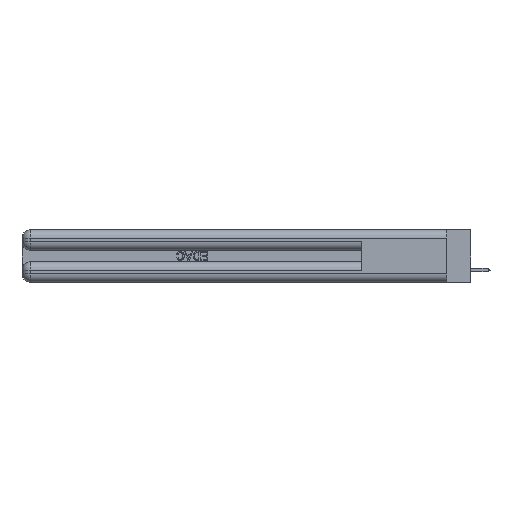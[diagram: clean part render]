
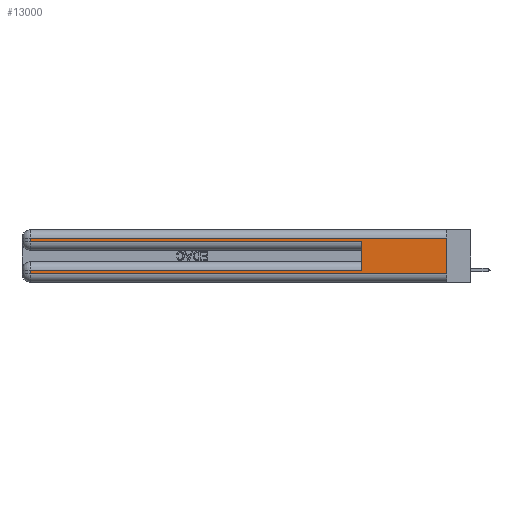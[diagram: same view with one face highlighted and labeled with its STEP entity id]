
A CAD part, left-side view. The second image highlights one B-rep face of the part: STEP entity #13000.
In plain terms, the highlighted planar face has unit normal (-1, 0, 0).
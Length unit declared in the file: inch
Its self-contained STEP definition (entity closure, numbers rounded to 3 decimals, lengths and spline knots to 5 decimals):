
#81 = ORIENTED_EDGE ( 'NONE', *, *, #29845, .T. ) ;
#892 = EDGE_LOOP ( 'NONE', ( #8477, #81, #23279, #6880, #42498, #15055, #4642, #9860 ) ) ;
#2024 = CARTESIAN_POINT ( 'NONE',  ( 0., 0., 0.085 ) ) ;
#2395 = CARTESIAN_POINT ( 'NONE',  ( 0., 2.94, 0.37 ) ) ;
#2813 = DIRECTION ( 'NONE',  ( 0., 0., -1. ) ) ;
#3315 = EDGE_CURVE ( 'NONE', #30173, #13856, #27101, .T. ) ;
#3468 = VECTOR ( 'NONE', #44397, 39.37008 ) ;
#4642 = ORIENTED_EDGE ( 'NONE', *, *, #40143, .T. ) ;
#6114 = LINE ( 'NONE', #21808, #14335 ) ;
#6879 = VERTEX_POINT ( 'NONE', #12419 ) ;
#6880 = ORIENTED_EDGE ( 'NONE', *, *, #42043, .T. ) ;
#7465 = AXIS2_PLACEMENT_3D ( 'NONE', #35042, #13983, #31778 ) ;
#7530 = VERTEX_POINT ( 'NONE', #21497 ) ;
#7731 = FACE_OUTER_BOUND ( 'NONE', #892, .T. ) ;
#8477 = ORIENTED_EDGE ( 'NONE', *, *, #14296, .F. ) ;
#8882 = LINE ( 'NONE', #28672, #34735 ) ;
#9617 = CARTESIAN_POINT ( 'NONE',  ( 0., 0., 0.37 ) ) ;
#9860 = ORIENTED_EDGE ( 'NONE', *, *, #44880, .T. ) ;
#10630 = CARTESIAN_POINT ( 'NONE',  ( 0., 0., 0.31 ) ) ;
#10912 = LINE ( 'NONE', #16637, #25170 ) ;
#11363 = DIRECTION ( 'NONE',  ( 0., 1., 0. ) ) ;
#12179 = CARTESIAN_POINT ( 'NONE',  ( 0., 2.94, 0.37 ) ) ;
#12419 = CARTESIAN_POINT ( 'NONE',  ( 0., 2.94, 0.06 ) ) ;
#13000 = ADVANCED_FACE ( 'NONE', ( #7731 ), #27669, .F. ) ;
#13856 = VERTEX_POINT ( 'NONE', #17220 ) ;
#13983 = DIRECTION ( 'NONE',  ( 1., 0., 0. ) ) ;
#14296 = EDGE_CURVE ( 'NONE', #29142, #7530, #25715, .T. ) ;
#14335 = VECTOR ( 'NONE', #11363, 39.37008 ) ;
#15055 = ORIENTED_EDGE ( 'NONE', *, *, #3315, .T. ) ;
#15820 = VECTOR ( 'NONE', #2813, 39.37008 ) ;
#16637 = CARTESIAN_POINT ( 'NONE',  ( 0., 0., 0.06 ) ) ;
#16802 = LINE ( 'NONE', #20202, #37574 ) ;
#17220 = CARTESIAN_POINT ( 'NONE',  ( 0., 2.94, 0.085 ) ) ;
#18384 = DIRECTION ( 'NONE',  ( 0., 0., 1. ) ) ;
#20202 = CARTESIAN_POINT ( 'NONE',  ( 0., 0., 0.285 ) ) ;
#20359 = DIRECTION ( 'NONE',  ( 0., 0., -1. ) ) ;
#21222 = VERTEX_POINT ( 'NONE', #44408 ) ;
#21497 = CARTESIAN_POINT ( 'NONE',  ( 0., 0., 0.06 ) ) ;
#21632 = EDGE_CURVE ( 'NONE', #30173, #21222, #8882, .T. ) ;
#21808 = CARTESIAN_POINT ( 'NONE',  ( 0., 0., 0.31 ) ) ;
#23279 = ORIENTED_EDGE ( 'NONE', *, *, #43675, .T. ) ;
#25148 = CARTESIAN_POINT ( 'NONE',  ( 0., 0.6, 0.085 ) ) ;
#25170 = VECTOR ( 'NONE', #30914, 39.37008 ) ;
#25715 = LINE ( 'NONE', #9617, #15820 ) ;
#26306 = DIRECTION ( 'NONE',  ( 0., 1., 0. ) ) ;
#26422 = VERTEX_POINT ( 'NONE', #34368 ) ;
#27101 = LINE ( 'NONE', #2024, #29225 ) ;
#27669 = PLANE ( 'NONE',  #7465 ) ;
#28672 = CARTESIAN_POINT ( 'NONE',  ( 0., 0.6, 0.145 ) ) ;
#29142 = VERTEX_POINT ( 'NONE', #10630 ) ;
#29225 = VECTOR ( 'NONE', #26306, 39.37008 ) ;
#29845 = EDGE_CURVE ( 'NONE', #29142, #26422, #6114, .T. ) ;
#30173 = VERTEX_POINT ( 'NONE', #25148 ) ;
#30914 = DIRECTION ( 'NONE',  ( 0., -1., 0. ) ) ;
#31778 = DIRECTION ( 'NONE',  ( 0., 0., -1. ) ) ;
#31917 = VECTOR ( 'NONE', #20359, 39.37008 ) ;
#34368 = CARTESIAN_POINT ( 'NONE',  ( 0., 2.94, 0.31 ) ) ;
#34735 = VECTOR ( 'NONE', #18384, 39.37008 ) ;
#34869 = LINE ( 'NONE', #2395, #3468 ) ;
#35042 = CARTESIAN_POINT ( 'NONE',  ( 0., 0., 0.37 ) ) ;
#35536 = VERTEX_POINT ( 'NONE', #35828 ) ;
#35828 = CARTESIAN_POINT ( 'NONE',  ( 0., 2.94, 0.285 ) ) ;
#37574 = VECTOR ( 'NONE', #41447, 39.37008 ) ;
#40143 = EDGE_CURVE ( 'NONE', #13856, #6879, #34869, .T. ) ;
#41447 = DIRECTION ( 'NONE',  ( 0., -1., 0. ) ) ;
#42043 = EDGE_CURVE ( 'NONE', #35536, #21222, #16802, .T. ) ;
#42498 = ORIENTED_EDGE ( 'NONE', *, *, #21632, .F. ) ;
#43482 = LINE ( 'NONE', #12179, #31917 ) ;
#43675 = EDGE_CURVE ( 'NONE', #26422, #35536, #43482, .T. ) ;
#44397 = DIRECTION ( 'NONE',  ( 0., 0., -1. ) ) ;
#44408 = CARTESIAN_POINT ( 'NONE',  ( 0., 0.6, 0.285 ) ) ;
#44880 = EDGE_CURVE ( 'NONE', #6879, #7530, #10912, .T. ) ;
